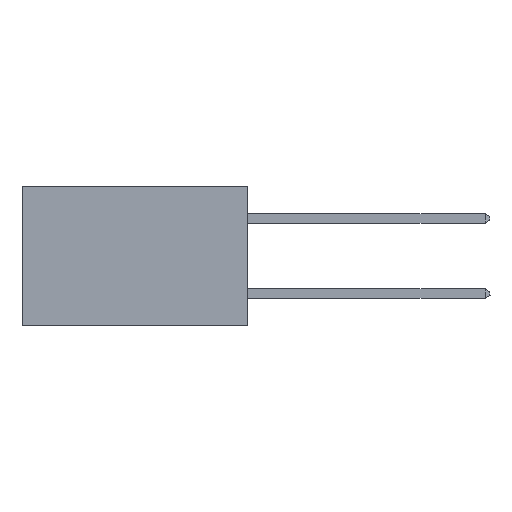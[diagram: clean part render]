
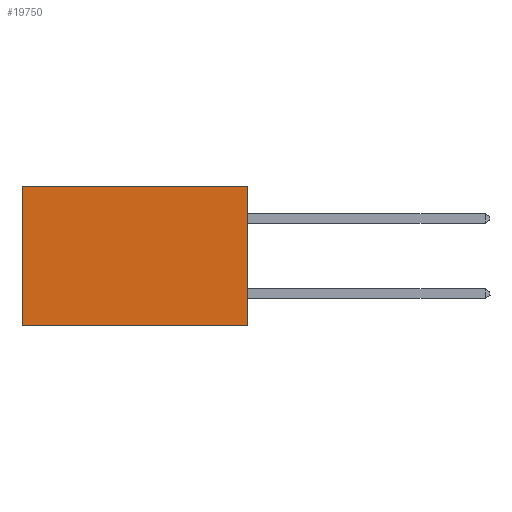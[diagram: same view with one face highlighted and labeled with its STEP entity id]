
A CAD part, left-side view. The second image highlights one B-rep face of the part: STEP entity #19750.
In plain terms, the highlighted planar face has unit normal (-1, 0, 0).
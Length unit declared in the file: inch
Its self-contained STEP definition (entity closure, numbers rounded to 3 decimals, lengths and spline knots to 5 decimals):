
#756 = CARTESIAN_POINT ( 'NONE',  ( 0.298, 0.6, -0.37 ) ) ;
#1592 = VERTEX_POINT ( 'NONE', #15253 ) ;
#2538 = VERTEX_POINT ( 'NONE', #8449 ) ;
#3582 = EDGE_CURVE ( 'NONE', #2538, #6493, #17124, .T. ) ;
#3688 = VECTOR ( 'NONE', #9300, 39.37008 ) ;
#4897 = ORIENTED_EDGE ( 'NONE', *, *, #20840, .F. ) ;
#5044 = LINE ( 'NONE', #22677, #25190 ) ;
#5329 = PLANE ( 'NONE',  #17741 ) ;
#6324 = VECTOR ( 'NONE', #19613, 39.37008 ) ;
#6493 = VERTEX_POINT ( 'NONE', #756 ) ;
#7347 = CARTESIAN_POINT ( 'NONE',  ( 0.298, 0., 0. ) ) ;
#7580 = EDGE_CURVE ( 'NONE', #7740, #1592, #24862, .T. ) ;
#7740 = VERTEX_POINT ( 'NONE', #10665 ) ;
#8449 = CARTESIAN_POINT ( 'NONE',  ( 0.298, 0., -0.37 ) ) ;
#9204 = CARTESIAN_POINT ( 'NONE',  ( 0.298, 0., -0.37 ) ) ;
#9300 = DIRECTION ( 'NONE',  ( 0., 1., 0. ) ) ;
#9396 = DIRECTION ( 'NONE',  ( 1., 0., 0. ) ) ;
#10115 = DIRECTION ( 'NONE',  ( 0., 0., -1. ) ) ;
#10665 = CARTESIAN_POINT ( 'NONE',  ( 0.298, 0., 0. ) ) ;
#13430 = ORIENTED_EDGE ( 'NONE', *, *, #7580, .T. ) ;
#15253 = CARTESIAN_POINT ( 'NONE',  ( 0.298, 0.6, 0. ) ) ;
#15547 = DIRECTION ( 'NONE',  ( 0., 1., 0. ) ) ;
#16436 = ORIENTED_EDGE ( 'NONE', *, *, #23094, .T. ) ;
#17124 = LINE ( 'NONE', #9204, #3688 ) ;
#17432 = ORIENTED_EDGE ( 'NONE', *, *, #3582, .F. ) ;
#17741 = AXIS2_PLACEMENT_3D ( 'NONE', #7347, #9396, #23668 ) ;
#19338 = CARTESIAN_POINT ( 'NONE',  ( 0.298, 0., 0. ) ) ;
#19613 = DIRECTION ( 'NONE',  ( 0., 0., -1. ) ) ;
#19750 = ADVANCED_FACE ( 'NONE', ( #19860 ), #5329, .F. ) ;
#19860 = FACE_OUTER_BOUND ( 'NONE', #24634, .T. ) ;
#20840 = EDGE_CURVE ( 'NONE', #7740, #2538, #25528, .T. ) ;
#22006 = VECTOR ( 'NONE', #15547, 39.37008 ) ;
#22677 = CARTESIAN_POINT ( 'NONE',  ( 0.298, 0.6, 0. ) ) ;
#23094 = EDGE_CURVE ( 'NONE', #1592, #6493, #5044, .T. ) ;
#23668 = DIRECTION ( 'NONE',  ( 0., 0., -1. ) ) ;
#24634 = EDGE_LOOP ( 'NONE', ( #16436, #17432, #4897, #13430 ) ) ;
#24862 = LINE ( 'NONE', #25293, #22006 ) ;
#25190 = VECTOR ( 'NONE', #10115, 39.37008 ) ;
#25293 = CARTESIAN_POINT ( 'NONE',  ( 0.298, 0., 0. ) ) ;
#25528 = LINE ( 'NONE', #19338, #6324 ) ;
